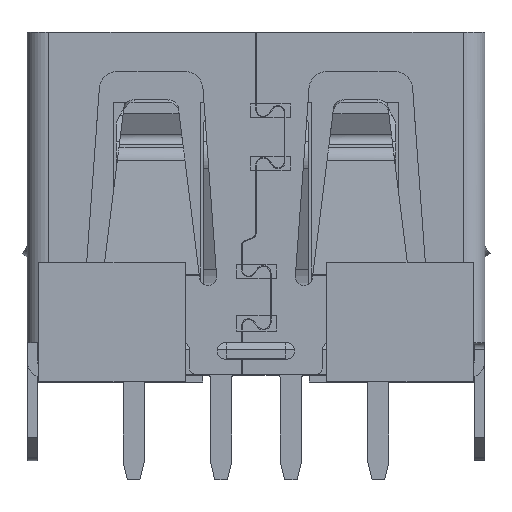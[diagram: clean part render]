
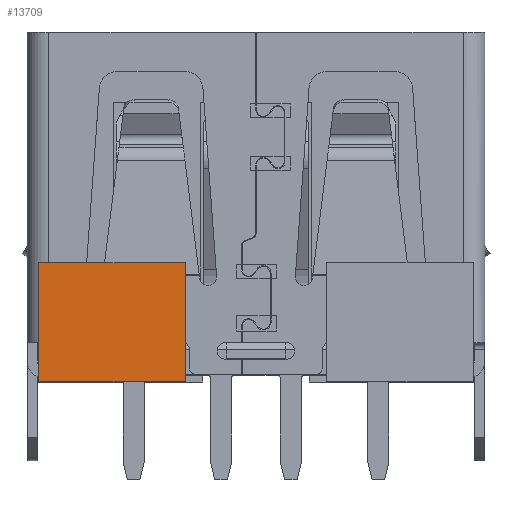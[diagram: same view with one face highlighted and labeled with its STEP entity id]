
A CAD part, top view. The second image highlights one B-rep face of the part: STEP entity #13709.
In plain terms, the highlighted planar face has unit normal (0, 0, 1).
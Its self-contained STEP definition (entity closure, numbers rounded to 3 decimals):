
#822 = EDGE_CURVE ( 'NONE', #22414, #22173, #11940, .T. ) ;
#1926 = VECTOR ( 'NONE', #25815, 1000. ) ;
#2511 = EDGE_CURVE ( 'NONE', #24512, #8773, #15224, .T. ) ;
#2844 = LINE ( 'NONE', #25397, #25739 ) ;
#2892 = DIRECTION ( 'NONE',  ( 0., 1., 0. ) ) ;
#3501 = AXIS2_PLACEMENT_3D ( 'NONE', #13146, #21381, #2892 ) ;
#3957 = CARTESIAN_POINT ( 'NONE',  ( -6.221, 0.452, 4.666 ) ) ;
#5935 = VECTOR ( 'NONE', #6724, 1000. ) ;
#6548 = CARTESIAN_POINT ( 'NONE',  ( -6.221, -2.948, 4.666 ) ) ;
#6724 = DIRECTION ( 'NONE',  ( 0., -1., 0. ) ) ;
#7099 = EDGE_CURVE ( 'NONE', #8773, #22173, #15400, .T. ) ;
#8773 = VERTEX_POINT ( 'NONE', #12005 ) ;
#9154 = CARTESIAN_POINT ( 'NONE',  ( -2.021, -1.248, 4.666 ) ) ;
#9157 = CARTESIAN_POINT ( 'NONE',  ( -2.021, 0.452, 4.666 ) ) ;
#9906 = DIRECTION ( 'NONE',  ( 0., -1., 0. ) ) ;
#10989 = ORIENTED_EDGE ( 'NONE', *, *, #822, .T. ) ;
#11940 = LINE ( 'NONE', #20169, #19404 ) ;
#12005 = CARTESIAN_POINT ( 'NONE',  ( -2.021, -2.948, 4.666 ) ) ;
#13146 = CARTESIAN_POINT ( 'NONE',  ( -4.121, -1.248, 4.666 ) ) ;
#13709 = ADVANCED_FACE ( 'NONE', ( #15161 ), #23422, .F. ) ;
#14586 = EDGE_LOOP ( 'NONE', ( #19113, #10989, #26155, #20762 ) ) ;
#15161 = FACE_OUTER_BOUND ( 'NONE', #14586, .T. ) ;
#15224 = LINE ( 'NONE', #9154, #5935 ) ;
#15400 = LINE ( 'NONE', #23664, #1926 ) ;
#19113 = ORIENTED_EDGE ( 'NONE', *, *, #21427, .F. ) ;
#19404 = VECTOR ( 'NONE', #9906, 1000. ) ;
#20169 = CARTESIAN_POINT ( 'NONE',  ( -6.221, -1.248, 4.666 ) ) ;
#20762 = ORIENTED_EDGE ( 'NONE', *, *, #2511, .F. ) ;
#21381 = DIRECTION ( 'NONE',  ( 0., 0., -1. ) ) ;
#21427 = EDGE_CURVE ( 'NONE', #22414, #24512, #2844, .T. ) ;
#21610 = DIRECTION ( 'NONE',  ( 1., 0., 0. ) ) ;
#22173 = VERTEX_POINT ( 'NONE', #6548 ) ;
#22414 = VERTEX_POINT ( 'NONE', #3957 ) ;
#23422 = PLANE ( 'NONE',  #3501 ) ;
#23664 = CARTESIAN_POINT ( 'NONE',  ( -4.121, -2.948, 4.666 ) ) ;
#24512 = VERTEX_POINT ( 'NONE', #9157 ) ;
#25397 = CARTESIAN_POINT ( 'NONE',  ( -4.121, 0.452, 4.666 ) ) ;
#25739 = VECTOR ( 'NONE', #21610, 1000. ) ;
#25815 = DIRECTION ( 'NONE',  ( -1., 0., 0. ) ) ;
#26155 = ORIENTED_EDGE ( 'NONE', *, *, #7099, .F. ) ;
